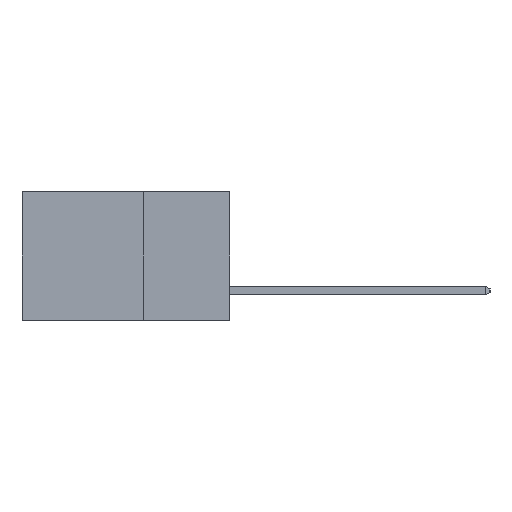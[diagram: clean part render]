
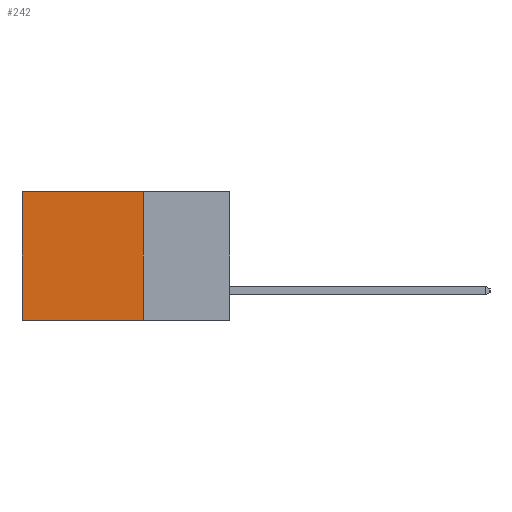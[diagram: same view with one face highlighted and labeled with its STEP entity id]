
A CAD part, left-side view. The second image highlights one B-rep face of the part: STEP entity #242.
In plain terms, the highlighted planar face has unit normal (-1, 0, 0).
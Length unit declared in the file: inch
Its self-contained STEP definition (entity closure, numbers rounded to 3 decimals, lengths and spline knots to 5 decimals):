
#135 = CARTESIAN_POINT ( 'NONE',  ( 0.298, 0.6, -0.37 ) ) ;
#242 = ADVANCED_FACE ( 'NONE', ( #3178 ), #5509, .F. ) ;
#613 = VECTOR ( 'NONE', #4434, 39.37008 ) ;
#648 = DIRECTION ( 'NONE',  ( 0., 0., -1. ) ) ;
#886 = CARTESIAN_POINT ( 'NONE',  ( 0.298, 0.25, 0. ) ) ;
#1109 = EDGE_CURVE ( 'NONE', #5684, #8296, #5259, .T. ) ;
#2416 = CARTESIAN_POINT ( 'NONE',  ( 0.298, 0.25, 0. ) ) ;
#2424 = ORIENTED_EDGE ( 'NONE', *, *, #10816, .T. ) ;
#2558 = DIRECTION ( 'NONE',  ( 0., 0., -1. ) ) ;
#2601 = LINE ( 'NONE', #7268, #7089 ) ;
#2632 = ORIENTED_EDGE ( 'NONE', *, *, #1109, .F. ) ;
#2644 = ORIENTED_EDGE ( 'NONE', *, *, #5109, .F. ) ;
#2656 = EDGE_CURVE ( 'NONE', #10131, #2957, #5773, .T. ) ;
#2664 = ORIENTED_EDGE ( 'NONE', *, *, #2656, .T. ) ;
#2957 = VERTEX_POINT ( 'NONE', #3929 ) ;
#3178 = FACE_OUTER_BOUND ( 'NONE', #6424, .T. ) ;
#3929 = CARTESIAN_POINT ( 'NONE',  ( 0.298, 0.6, 0. ) ) ;
#3943 = DIRECTION ( 'NONE',  ( 1., 0., 0. ) ) ;
#4434 = DIRECTION ( 'NONE',  ( 0., 1., 0. ) ) ;
#5109 = EDGE_CURVE ( 'NONE', #10131, #5684, #7473, .T. ) ;
#5259 = LINE ( 'NONE', #5847, #7545 ) ;
#5509 = PLANE ( 'NONE',  #11547 ) ;
#5684 = VERTEX_POINT ( 'NONE', #8395 ) ;
#5773 = LINE ( 'NONE', #6583, #613 ) ;
#5847 = CARTESIAN_POINT ( 'NONE',  ( 0.298, 0.25, -0.37 ) ) ;
#6424 = EDGE_LOOP ( 'NONE', ( #2424, #2632, #2644, #2664 ) ) ;
#6583 = CARTESIAN_POINT ( 'NONE',  ( 0.298, 0.25, 0. ) ) ;
#7089 = VECTOR ( 'NONE', #648, 39.37008 ) ;
#7268 = CARTESIAN_POINT ( 'NONE',  ( 0.298, 0.6, 0. ) ) ;
#7400 = CARTESIAN_POINT ( 'NONE',  ( 0.298, 0.25, 0. ) ) ;
#7473 = LINE ( 'NONE', #2416, #9865 ) ;
#7545 = VECTOR ( 'NONE', #11423, 39.37008 ) ;
#8296 = VERTEX_POINT ( 'NONE', #135 ) ;
#8395 = CARTESIAN_POINT ( 'NONE',  ( 0.298, 0.25, -0.37 ) ) ;
#9865 = VECTOR ( 'NONE', #2558, 39.37008 ) ;
#10131 = VERTEX_POINT ( 'NONE', #7400 ) ;
#10363 = DIRECTION ( 'NONE',  ( 0., 0., -1. ) ) ;
#10816 = EDGE_CURVE ( 'NONE', #2957, #8296, #2601, .T. ) ;
#11423 = DIRECTION ( 'NONE',  ( 0., 1., 0. ) ) ;
#11547 = AXIS2_PLACEMENT_3D ( 'NONE', #886, #3943, #10363 ) ;
